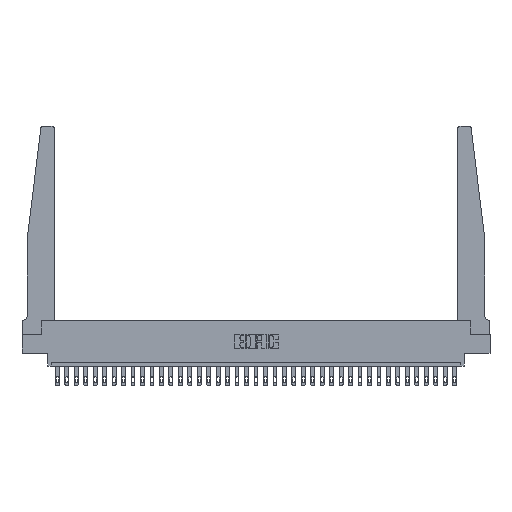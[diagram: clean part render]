
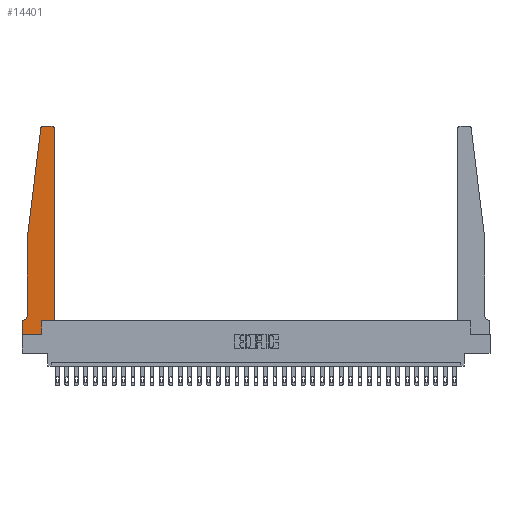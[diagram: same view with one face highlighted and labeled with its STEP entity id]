
A CAD part, top view. The second image highlights one B-rep face of the part: STEP entity #14401.
In plain terms, the highlighted planar face has unit normal (0, 0, 1).
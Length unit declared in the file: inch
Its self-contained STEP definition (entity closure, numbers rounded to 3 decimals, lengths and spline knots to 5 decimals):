
#158 = DIRECTION ( 'NONE',  ( 0., -1., 0. ) ) ;
#188 = EDGE_CURVE ( 'NONE', #13783, #2127, #23100, .T. ) ;
#884 = CARTESIAN_POINT ( 'NONE',  ( 0.25, 2.75, 0.37 ) ) ;
#998 = VERTEX_POINT ( 'NONE', #21187 ) ;
#1483 = CIRCLE ( 'NONE', #26160, 0.05 ) ;
#1891 = VERTEX_POINT ( 'NONE', #25633 ) ;
#2127 = VERTEX_POINT ( 'NONE', #9983 ) ;
#2203 = EDGE_CURVE ( 'NONE', #11007, #23411, #24655, .T. ) ;
#3343 = VECTOR ( 'NONE', #15268, 39.37008 ) ;
#3554 = CARTESIAN_POINT ( 'NONE',  ( 0.065, 0.2375, 0.37 ) ) ;
#3968 = DIRECTION ( 'NONE',  ( 1., 0., 0. ) ) ;
#4531 = EDGE_CURVE ( 'NONE', #10509, #13045, #5990, .T. ) ;
#4549 = CARTESIAN_POINT ( 'NONE',  ( 0., 0., 0.37 ) ) ;
#5637 = DIRECTION ( 'NONE',  ( 1., 0., 0. ) ) ;
#5883 = CARTESIAN_POINT ( 'NONE',  ( 0.425, 0.18, 0.37 ) ) ;
#5941 = DIRECTION ( 'NONE',  ( 0., 1., 0. ) ) ;
#5990 = LINE ( 'NONE', #28370, #9368 ) ;
#6286 = DIRECTION ( 'NONE',  ( -0.122, -0.992, 0. ) ) ;
#6405 = VECTOR ( 'NONE', #158, 39.37008 ) ;
#7084 = CARTESIAN_POINT ( 'NONE',  ( 0., 0.1875, 0.37 ) ) ;
#7401 = CARTESIAN_POINT ( 'NONE',  ( 0.065, 1.25, 0.37 ) ) ;
#7434 = ORIENTED_EDGE ( 'NONE', *, *, #10372, .T. ) ;
#8333 = EDGE_CURVE ( 'NONE', #1891, #998, #15988, .T. ) ;
#8412 = VECTOR ( 'NONE', #10390, 39.37008 ) ;
#8738 = CARTESIAN_POINT ( 'NONE',  ( 0.425, 0.18, 0.37 ) ) ;
#9368 = VECTOR ( 'NONE', #6286, 39.37008 ) ;
#9511 = PLANE ( 'NONE',  #10821 ) ;
#9572 = ORIENTED_EDGE ( 'NONE', *, *, #21852, .T. ) ;
#9683 = VERTEX_POINT ( 'NONE', #31064 ) ;
#9698 = CARTESIAN_POINT ( 'NONE',  ( 0.27653, 2.72, 0.37 ) ) ;
#9983 = CARTESIAN_POINT ( 'NONE',  ( 0., 0.1875, 0.37 ) ) ;
#10372 = EDGE_CURVE ( 'NONE', #23411, #9683, #28244, .T. ) ;
#10390 = DIRECTION ( 'NONE',  ( 0., -1., 0. ) ) ;
#10509 = VERTEX_POINT ( 'NONE', #17145 ) ;
#10821 = AXIS2_PLACEMENT_3D ( 'NONE', #7084, #19364, #5637 ) ;
#11007 = VERTEX_POINT ( 'NONE', #17266 ) ;
#11020 = VERTEX_POINT ( 'NONE', #27546 ) ;
#11259 = CARTESIAN_POINT ( 'NONE',  ( 0.2605, 0.18, 0.37 ) ) ;
#12050 = EDGE_CURVE ( 'NONE', #23924, #13783, #1483, .T. ) ;
#12612 = VECTOR ( 'NONE', #5941, 39.37008 ) ;
#12671 = LINE ( 'NONE', #22474, #8412 ) ;
#12674 = EDGE_CURVE ( 'NONE', #11020, #11007, #22278, .T. ) ;
#12908 = DIRECTION ( 'NONE',  ( 0., 0., 1. ) ) ;
#13045 = VERTEX_POINT ( 'NONE', #7401 ) ;
#13449 = DIRECTION ( 'NONE',  ( 1., 0., 0. ) ) ;
#13759 = CARTESIAN_POINT ( 'NONE',  ( 0.015, 0.1875, 0.37 ) ) ;
#13783 = VERTEX_POINT ( 'NONE', #13759 ) ;
#13955 = ORIENTED_EDGE ( 'NONE', *, *, #4531, .T. ) ;
#14401 = ADVANCED_FACE ( 'NONE', ( #31574 ), #9511, .T. ) ;
#15268 = DIRECTION ( 'NONE',  ( 0., 1., 0. ) ) ;
#15869 = DIRECTION ( 'NONE',  ( -1., 0., 0. ) ) ;
#15988 = CIRCLE ( 'NONE', #18491, 0.03 ) ;
#16564 = CARTESIAN_POINT ( 'NONE',  ( 0.395, 2.72, 0.37 ) ) ;
#16692 = ORIENTED_EDGE ( 'NONE', *, *, #27889, .T. ) ;
#17145 = CARTESIAN_POINT ( 'NONE',  ( 0.24675, 2.72367, 0.37 ) ) ;
#17266 = CARTESIAN_POINT ( 'NONE',  ( 0.2605, 0., 0.37 ) ) ;
#18137 = LINE ( 'NONE', #884, #30729 ) ;
#18491 = AXIS2_PLACEMENT_3D ( 'NONE', #16564, #23324, #3968 ) ;
#19364 = DIRECTION ( 'NONE',  ( 0., 0., 1. ) ) ;
#19551 = DIRECTION ( 'NONE',  ( 1., 0., 0. ) ) ;
#19621 = VECTOR ( 'NONE', #28385, 39.37008 ) ;
#19664 = CARTESIAN_POINT ( 'NONE',  ( 0.2605, 0.18, 0.37 ) ) ;
#20435 = CARTESIAN_POINT ( 'NONE',  ( 0.015, 0.2375, 0.37 ) ) ;
#20592 = VERTEX_POINT ( 'NONE', #30595 ) ;
#20932 = AXIS2_PLACEMENT_3D ( 'NONE', #9698, #12908, #19551 ) ;
#21170 = ORIENTED_EDGE ( 'NONE', *, *, #25541, .T. ) ;
#21187 = CARTESIAN_POINT ( 'NONE',  ( 0.395, 2.75, 0.37 ) ) ;
#21694 = ORIENTED_EDGE ( 'NONE', *, *, #8333, .T. ) ;
#21824 = ORIENTED_EDGE ( 'NONE', *, *, #188, .T. ) ;
#21852 = EDGE_CURVE ( 'NONE', #13045, #23924, #22056, .T. ) ;
#21959 = DIRECTION ( 'NONE',  ( 1., 0., 0. ) ) ;
#22056 = LINE ( 'NONE', #31380, #6405 ) ;
#22278 = LINE ( 'NONE', #4549, #26704 ) ;
#22474 = CARTESIAN_POINT ( 'NONE',  ( 0., 0., 0.37 ) ) ;
#23100 = LINE ( 'NONE', #23246, #19621 ) ;
#23246 = CARTESIAN_POINT ( 'NONE',  ( 0.065, 0.1875, 0.37 ) ) ;
#23324 = DIRECTION ( 'NONE',  ( 0., 0., 1. ) ) ;
#23411 = VERTEX_POINT ( 'NONE', #11259 ) ;
#23924 = VERTEX_POINT ( 'NONE', #3554 ) ;
#24242 = ORIENTED_EDGE ( 'NONE', *, *, #12050, .T. ) ;
#24655 = LINE ( 'NONE', #19664, #12612 ) ;
#25040 = CIRCLE ( 'NONE', #20932, 0.03 ) ;
#25145 = EDGE_LOOP ( 'NONE', ( #28701, #21170, #13955, #9572, #24242, #21824, #28122, #28540, #27648, #7434, #16692, #21694 ) ) ;
#25541 = EDGE_CURVE ( 'NONE', #20592, #10509, #25040, .T. ) ;
#25565 = DIRECTION ( 'NONE',  ( -1., 0., 0. ) ) ;
#25633 = CARTESIAN_POINT ( 'NONE',  ( 0.425, 2.72, 0.37 ) ) ;
#26160 = AXIS2_PLACEMENT_3D ( 'NONE', #20435, #29909, #25565 ) ;
#26429 = EDGE_CURVE ( 'NONE', #2127, #11020, #12671, .T. ) ;
#26704 = VECTOR ( 'NONE', #21959, 39.37008 ) ;
#27546 = CARTESIAN_POINT ( 'NONE',  ( 0., 0., 0.37 ) ) ;
#27648 = ORIENTED_EDGE ( 'NONE', *, *, #2203, .T. ) ;
#27889 = EDGE_CURVE ( 'NONE', #9683, #1891, #27963, .T. ) ;
#27963 = LINE ( 'NONE', #5883, #3343 ) ;
#28122 = ORIENTED_EDGE ( 'NONE', *, *, #26429, .T. ) ;
#28244 = LINE ( 'NONE', #8738, #31649 ) ;
#28370 = CARTESIAN_POINT ( 'NONE',  ( 0.065, 1.25, 0.37 ) ) ;
#28385 = DIRECTION ( 'NONE',  ( -1., 0., 0. ) ) ;
#28540 = ORIENTED_EDGE ( 'NONE', *, *, #12674, .T. ) ;
#28701 = ORIENTED_EDGE ( 'NONE', *, *, #31474, .T. ) ;
#29909 = DIRECTION ( 'NONE',  ( 0., 0., -1. ) ) ;
#30595 = CARTESIAN_POINT ( 'NONE',  ( 0.27653, 2.75, 0.37 ) ) ;
#30729 = VECTOR ( 'NONE', #15869, 39.37008 ) ;
#31064 = CARTESIAN_POINT ( 'NONE',  ( 0.425, 0.18, 0.37 ) ) ;
#31380 = CARTESIAN_POINT ( 'NONE',  ( 0.065, 1.25, 0.37 ) ) ;
#31474 = EDGE_CURVE ( 'NONE', #998, #20592, #18137, .T. ) ;
#31574 = FACE_OUTER_BOUND ( 'NONE', #25145, .T. ) ;
#31649 = VECTOR ( 'NONE', #13449, 39.37008 ) ;
